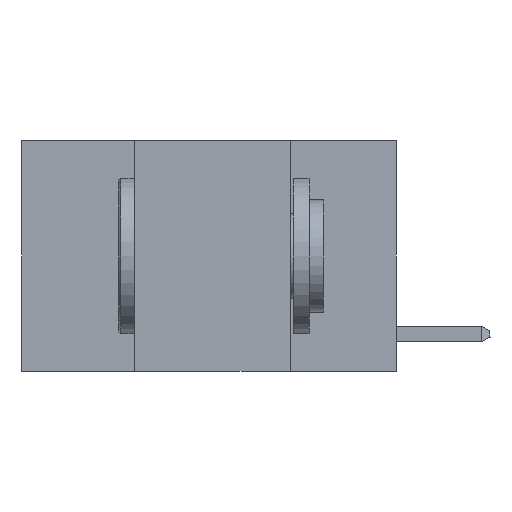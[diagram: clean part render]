
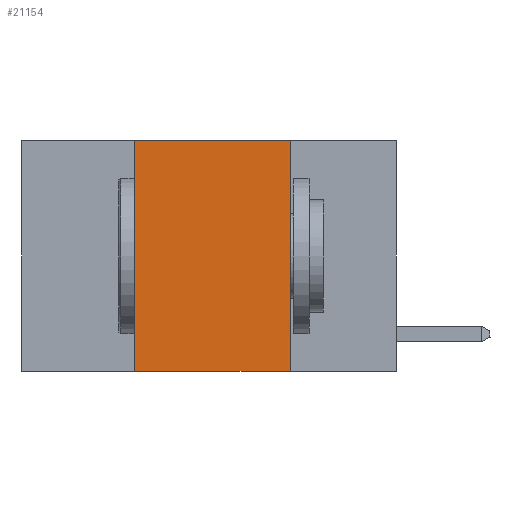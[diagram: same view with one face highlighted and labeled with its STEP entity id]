
A CAD part, left-side view. The second image highlights one B-rep face of the part: STEP entity #21154.
In plain terms, the highlighted planar face has unit normal (-1, 0, 0).
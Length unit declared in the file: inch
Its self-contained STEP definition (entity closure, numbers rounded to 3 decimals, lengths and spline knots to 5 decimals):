
#624 = CARTESIAN_POINT ( 'NONE',  ( 0., 0.42, 0. ) ) ;
#1501 = VERTEX_POINT ( 'NONE', #4017 ) ;
#3759 = EDGE_CURVE ( 'NONE', #23418, #25839, #27366, .T. ) ;
#4017 = CARTESIAN_POINT ( 'NONE',  ( 0., 0.17, -0.37 ) ) ;
#4460 = ORIENTED_EDGE ( 'NONE', *, *, #3759, .F. ) ;
#5465 = EDGE_CURVE ( 'NONE', #25839, #17341, #21796, .T. ) ;
#5471 = DIRECTION ( 'NONE',  ( 0., 0., 1. ) ) ;
#5906 = DIRECTION ( 'NONE',  ( 0., 0., -1. ) ) ;
#8347 = AXIS2_PLACEMENT_3D ( 'NONE', #10398, #29238, #5906 ) ;
#8411 = DIRECTION ( 'NONE',  ( 0., -1., 0. ) ) ;
#10282 = CARTESIAN_POINT ( 'NONE',  ( 0., 0.42, -0.37 ) ) ;
#10398 = CARTESIAN_POINT ( 'NONE',  ( 0., 0.6, 0. ) ) ;
#10825 = CARTESIAN_POINT ( 'NONE',  ( 0., 0.42, 0. ) ) ;
#11965 = CARTESIAN_POINT ( 'NONE',  ( 0., 0.17, 0. ) ) ;
#12067 = VECTOR ( 'NONE', #5471, 39.37008 ) ;
#12237 = VECTOR ( 'NONE', #18341, 39.37008 ) ;
#15806 = LINE ( 'NONE', #11965, #21670 ) ;
#16523 = DIRECTION ( 'NONE',  ( 0., 0., -1. ) ) ;
#16535 = ORIENTED_EDGE ( 'NONE', *, *, #5465, .F. ) ;
#17341 = VERTEX_POINT ( 'NONE', #24034 ) ;
#17533 = PLANE ( 'NONE',  #8347 ) ;
#18341 = DIRECTION ( 'NONE',  ( 0., -1., 0. ) ) ;
#18646 = EDGE_CURVE ( 'NONE', #23418, #1501, #24261, .T. ) ;
#19447 = EDGE_CURVE ( 'NONE', #17341, #1501, #15806, .T. ) ;
#21154 = ADVANCED_FACE ( 'NONE', ( #27362 ), #17533, .F. ) ;
#21670 = VECTOR ( 'NONE', #16523, 39.37008 ) ;
#21796 = LINE ( 'NONE', #24695, #29789 ) ;
#23418 = VERTEX_POINT ( 'NONE', #10282 ) ;
#24034 = CARTESIAN_POINT ( 'NONE',  ( 0., 0.17, 0. ) ) ;
#24261 = LINE ( 'NONE', #29744, #12237 ) ;
#24695 = CARTESIAN_POINT ( 'NONE',  ( 0., 0.6, 0. ) ) ;
#25839 = VERTEX_POINT ( 'NONE', #10825 ) ;
#26874 = ORIENTED_EDGE ( 'NONE', *, *, #18646, .T. ) ;
#27362 = FACE_OUTER_BOUND ( 'NONE', #29423, .T. ) ;
#27366 = LINE ( 'NONE', #624, #12067 ) ;
#28724 = ORIENTED_EDGE ( 'NONE', *, *, #19447, .F. ) ;
#29238 = DIRECTION ( 'NONE',  ( 1., 0., 0. ) ) ;
#29423 = EDGE_LOOP ( 'NONE', ( #28724, #16535, #4460, #26874 ) ) ;
#29744 = CARTESIAN_POINT ( 'NONE',  ( 0., 0.6, -0.37 ) ) ;
#29789 = VECTOR ( 'NONE', #8411, 39.37008 ) ;
